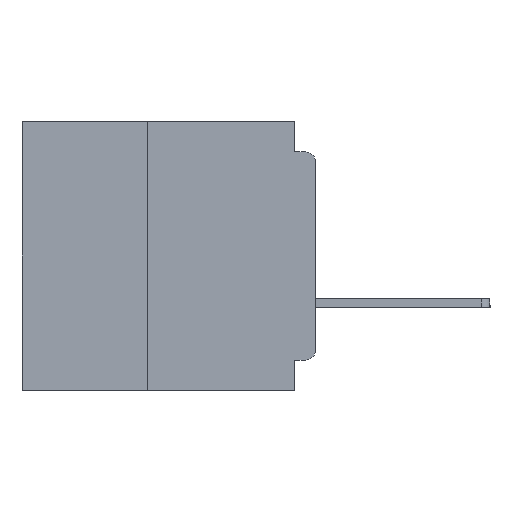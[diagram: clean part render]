
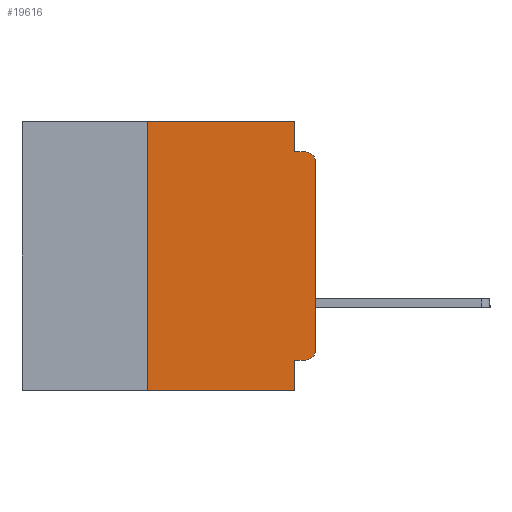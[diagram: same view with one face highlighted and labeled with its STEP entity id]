
A CAD part, left-side view. The second image highlights one B-rep face of the part: STEP entity #19616.
In plain terms, the highlighted planar face has unit normal (-1, 0, 0).
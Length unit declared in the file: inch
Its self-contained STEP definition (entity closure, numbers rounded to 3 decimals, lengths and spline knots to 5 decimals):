
#443 = EDGE_CURVE ( 'NONE', #21860, #24213, #23491, .T. ) ;
#449 = VECTOR ( 'NONE', #14257, 39.37008 ) ;
#522 = EDGE_CURVE ( 'NONE', #13965, #37571, #2747, .T. ) ;
#2244 = DIRECTION ( 'NONE',  ( 0., 1., 0. ) ) ;
#2320 = ORIENTED_EDGE ( 'NONE', *, *, #19561, .F. ) ;
#2747 = LINE ( 'NONE', #10587, #449 ) ;
#3349 = AXIS2_PLACEMENT_3D ( 'NONE', #23511, #9062, #34772 ) ;
#3452 = FACE_OUTER_BOUND ( 'NONE', #37102, .T. ) ;
#3478 = CARTESIAN_POINT ( 'NONE',  ( 0., 0.031, -0.4 ) ) ;
#4579 = ORIENTED_EDGE ( 'NONE', *, *, #32436, .F. ) ;
#5255 = CARTESIAN_POINT ( 'NONE',  ( 0., 0., -0.355 ) ) ;
#5793 = VECTOR ( 'NONE', #34462, 39.37008 ) ;
#6907 = CARTESIAN_POINT ( 'NONE',  ( 0., 0.031, -0.4 ) ) ;
#8774 = CARTESIAN_POINT ( 'NONE',  ( 0., 0.015, -0.06 ) ) ;
#8905 = VERTEX_POINT ( 'NONE', #42882 ) ;
#9062 = DIRECTION ( 'NONE',  ( 1., 0., 0. ) ) ;
#9425 = EDGE_CURVE ( 'NONE', #40155, #8905, #38046, .T. ) ;
#10394 = DIRECTION ( 'NONE',  ( -1., 0., 0. ) ) ;
#10587 = CARTESIAN_POINT ( 'NONE',  ( 0., 0.031, 0. ) ) ;
#12462 = DIRECTION ( 'NONE',  ( 0., 0., -1. ) ) ;
#13558 = VECTOR ( 'NONE', #25502, 39.37008 ) ;
#13965 = VERTEX_POINT ( 'NONE', #41044 ) ;
#14257 = DIRECTION ( 'NONE',  ( 0., 0., -1. ) ) ;
#15334 = ORIENTED_EDGE ( 'NONE', *, *, #522, .F. ) ;
#16617 = EDGE_CURVE ( 'NONE', #38533, #40838, #18182, .T. ) ;
#17022 = VECTOR ( 'NONE', #35498, 39.37008 ) ;
#17195 = CARTESIAN_POINT ( 'NONE',  ( 0., 0.015, -0.045 ) ) ;
#17532 = VECTOR ( 'NONE', #41923, 39.37008 ) ;
#17711 = CIRCLE ( 'NONE', #22090, 0.015 ) ;
#18035 = ORIENTED_EDGE ( 'NONE', *, *, #443, .F. ) ;
#18182 = LINE ( 'NONE', #31768, #17022 ) ;
#19561 = EDGE_CURVE ( 'NONE', #8905, #13965, #44762, .T. ) ;
#19616 = ADVANCED_FACE ( 'NONE', ( #3452 ), #45532, .F. ) ;
#19962 = LINE ( 'NONE', #42833, #28573 ) ;
#21860 = VERTEX_POINT ( 'NONE', #22906 ) ;
#21953 = EDGE_CURVE ( 'NONE', #40838, #30308, #17711, .T. ) ;
#22076 = CARTESIAN_POINT ( 'NONE',  ( 0., 0., -0.06 ) ) ;
#22090 = AXIS2_PLACEMENT_3D ( 'NONE', #8774, #34470, #12462 ) ;
#22906 = CARTESIAN_POINT ( 'NONE',  ( 0., 0.015, -0.355 ) ) ;
#23491 = LINE ( 'NONE', #5255, #41790 ) ;
#23511 = CARTESIAN_POINT ( 'NONE',  ( 0., 0.437, 0. ) ) ;
#24213 = VERTEX_POINT ( 'NONE', #25668 ) ;
#24631 = DIRECTION ( 'NONE',  ( 0., -1., 0. ) ) ;
#24929 = DIRECTION ( 'NONE',  ( 0., 0., 1. ) ) ;
#25162 = ORIENTED_EDGE ( 'NONE', *, *, #40511, .T. ) ;
#25502 = DIRECTION ( 'NONE',  ( 0., 0., -1. ) ) ;
#25668 = CARTESIAN_POINT ( 'NONE',  ( 0., 0.031, -0.355 ) ) ;
#25959 = ORIENTED_EDGE ( 'NONE', *, *, #40089, .T. ) ;
#27047 = CARTESIAN_POINT ( 'NONE',  ( 0., 0.437, 0. ) ) ;
#28573 = VECTOR ( 'NONE', #24631, 39.37008 ) ;
#28621 = CARTESIAN_POINT ( 'NONE',  ( 0., 0.25, -0.4 ) ) ;
#28999 = CARTESIAN_POINT ( 'NONE',  ( 0., 0.25, -0.4 ) ) ;
#30308 = VERTEX_POINT ( 'NONE', #17195 ) ;
#31007 = ORIENTED_EDGE ( 'NONE', *, *, #16617, .T. ) ;
#31631 = CARTESIAN_POINT ( 'NONE',  ( 0., 0.031, -0.045 ) ) ;
#31768 = CARTESIAN_POINT ( 'NONE',  ( 0., 0., 0. ) ) ;
#32379 = CARTESIAN_POINT ( 'NONE',  ( 0., 0.015, -0.34 ) ) ;
#32436 = EDGE_CURVE ( 'NONE', #37571, #30308, #19962, .T. ) ;
#33276 = EDGE_CURVE ( 'NONE', #24213, #37027, #42753, .T. ) ;
#34055 = ORIENTED_EDGE ( 'NONE', *, *, #21953, .T. ) ;
#34462 = DIRECTION ( 'NONE',  ( 0., -1., 0. ) ) ;
#34470 = DIRECTION ( 'NONE',  ( -1., 0., 0. ) ) ;
#34772 = DIRECTION ( 'NONE',  ( 0., 0., -1. ) ) ;
#35498 = DIRECTION ( 'NONE',  ( 0., 0., 1. ) ) ;
#36073 = DIRECTION ( 'NONE',  ( 0., 0., -1. ) ) ;
#36915 = VECTOR ( 'NONE', #24929, 39.37008 ) ;
#37027 = VERTEX_POINT ( 'NONE', #6907 ) ;
#37102 = EDGE_LOOP ( 'NONE', ( #31007, #34055, #4579, #15334, #2320, #41862, #25162, #44182, #18035, #25959 ) ) ;
#37571 = VERTEX_POINT ( 'NONE', #31631 ) ;
#37961 = CARTESIAN_POINT ( 'NONE',  ( 0., 0., -0.34 ) ) ;
#38046 = LINE ( 'NONE', #28621, #36915 ) ;
#38533 = VERTEX_POINT ( 'NONE', #37961 ) ;
#40089 = EDGE_CURVE ( 'NONE', #21860, #38533, #43305, .T. ) ;
#40155 = VERTEX_POINT ( 'NONE', #28999 ) ;
#40511 = EDGE_CURVE ( 'NONE', #40155, #37027, #45053, .T. ) ;
#40838 = VERTEX_POINT ( 'NONE', #22076 ) ;
#41044 = CARTESIAN_POINT ( 'NONE',  ( 0., 0.031, 0. ) ) ;
#41351 = AXIS2_PLACEMENT_3D ( 'NONE', #32379, #10394, #36073 ) ;
#41790 = VECTOR ( 'NONE', #2244, 39.37008 ) ;
#41862 = ORIENTED_EDGE ( 'NONE', *, *, #9425, .F. ) ;
#41923 = DIRECTION ( 'NONE',  ( 0., -1., 0. ) ) ;
#42753 = LINE ( 'NONE', #3478, #13558 ) ;
#42833 = CARTESIAN_POINT ( 'NONE',  ( 0., 0., -0.045 ) ) ;
#42882 = CARTESIAN_POINT ( 'NONE',  ( 0., 0.25, 0. ) ) ;
#43305 = CIRCLE ( 'NONE', #41351, 0.015 ) ;
#44182 = ORIENTED_EDGE ( 'NONE', *, *, #33276, .F. ) ;
#44762 = LINE ( 'NONE', #27047, #5793 ) ;
#45053 = LINE ( 'NONE', #45567, #17532 ) ;
#45532 = PLANE ( 'NONE',  #3349 ) ;
#45567 = CARTESIAN_POINT ( 'NONE',  ( 0., 0.437, -0.4 ) ) ;
